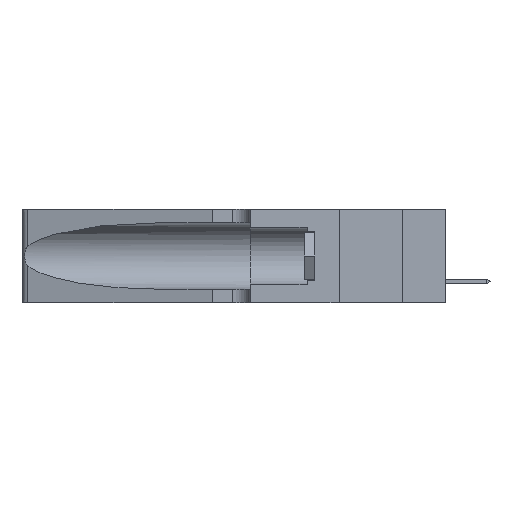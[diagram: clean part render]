
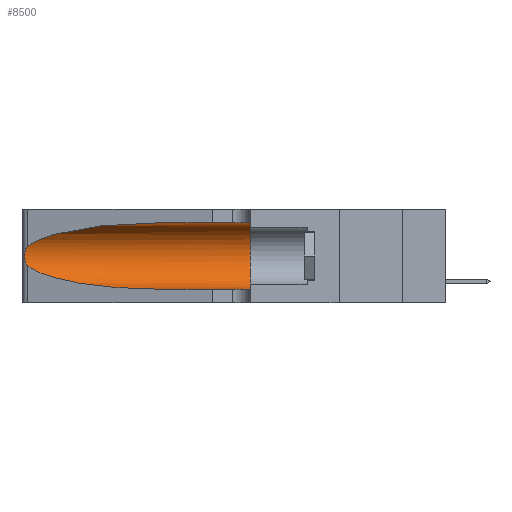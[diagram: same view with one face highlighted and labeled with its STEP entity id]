
A CAD part, left-side view. The second image highlights one B-rep face of the part: STEP entity #8500.
In plain terms, the highlighted cylindrical face has radius 3.308 mm (diameter 6.617 mm), a partial arc.
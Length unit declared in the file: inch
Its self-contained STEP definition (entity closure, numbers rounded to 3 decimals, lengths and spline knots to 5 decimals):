
#528 = ORIENTED_EDGE ( 'NONE', *, *, #15611, .F. ) ;
#548 = CARTESIAN_POINT ( 'NONE',  ( 0.1305, 1.61858, 0.185 ) ) ;
#616 = DIRECTION ( 'NONE',  ( 0., 0., -1. ) ) ;
#935 = CARTESIAN_POINT ( 'NONE',  ( 0.18966, 0.96281, 0.31525 ) ) ;
#961 = VECTOR ( 'NONE', #18069, 39.37008 ) ;
#1179 = CARTESIAN_POINT ( 'NONE',  ( 0.1305, 0.72297, 0.05475 ) ) ;
#1210 = AXIS2_PLACEMENT_3D ( 'NONE', #4689, #4761, #4612 ) ;
#1320 = CARTESIAN_POINT ( 'NONE',  ( 0.2373, 1.15595, 0.08982 ) ) ;
#1680 = CARTESIAN_POINT ( 'NONE',  ( 0.25487, 1.22718, 0.14631 ) ) ;
#1743 = VERTEX_POINT ( 'NONE', #8380 ) ;
#1961 = CARTESIAN_POINT ( 'NONE',  ( 0.25639, 1.23186, 0.15144 ) ) ;
#1983 = VERTEX_POINT ( 'NONE', #3956 ) ;
#2383 = B_SPLINE_CURVE_WITH_KNOTS ( 'NONE', 3,
 ( #12858, #4500, #4574, #17591, #7677, #8180, #15248, #16897, #18628, #20297, #18337, #1961, #13658, #1680 ),
 .UNSPECIFIED., .F., .F.,
 ( 4, 2, 2, 2, 2, 2, 4 ),
 ( 0., 0.00027, 0.00053, 0.00107, 0.0016, 0.00187, 0.00214 ),
 .UNSPECIFIED. ) ;
#2497 = VERTEX_POINT ( 'NONE', #15353 ) ;
#2686 = ORIENTED_EDGE ( 'NONE', *, *, #20262, .T. ) ;
#3001 = LINE ( 'NONE', #6966, #21076 ) ;
#3138 = ORIENTED_EDGE ( 'NONE', *, *, #20969, .T. ) ;
#3919 = ORIENTED_EDGE ( 'NONE', *, *, #8436, .F. ) ;
#3956 = CARTESIAN_POINT ( 'NONE',  ( 0.1305, 0.35, 0.31525 ) ) ;
#4019 = CIRCLE ( 'NONE', #1210, 0.13025 ) ;
#4206 = CARTESIAN_POINT ( 'NONE',  ( 0.25487, 1.22718, 0.22369 ) ) ;
#4500 = CARTESIAN_POINT ( 'NONE',  ( 0.25555, 1.22994, 0.2215 ) ) ;
#4574 = CARTESIAN_POINT ( 'NONE',  ( 0.25639, 1.23184, 0.21858 ) ) ;
#4578 = CARTESIAN_POINT ( 'NONE',  ( 0.18966, 0.96281, 0.05475 ) ) ;
#4612 = DIRECTION ( 'NONE',  ( 0., 0., 1. ) ) ;
#4689 = CARTESIAN_POINT ( 'NONE',  ( 0.1305, 0.35, 0.185 ) ) ;
#4761 = DIRECTION ( 'NONE',  ( 0., 1., 0. ) ) ;
#5115 = AXIS2_PLACEMENT_3D ( 'NONE', #548, #10481, #616 ) ;
#5933 = ORIENTED_EDGE ( 'NONE', *, *, #20416, .T. ) ;
#6376 = CARTESIAN_POINT ( 'NONE',  ( 0.1305, 1.61858, 0.05475 ) ) ;
#6966 = CARTESIAN_POINT ( 'NONE',  ( 0.1305, 1.61858, 0.31525 ) ) ;
#7677 = CARTESIAN_POINT ( 'NONE',  ( 0.25854, 1.2359, 0.20912 ) ) ;
#8180 = CARTESIAN_POINT ( 'NONE',  ( 0.26018, 1.23835, 0.19895 ) ) ;
#8380 = CARTESIAN_POINT ( 'NONE',  ( 0.1305, 0.72297, 0.31525 ) ) ;
#8436 = EDGE_CURVE ( 'NONE', #1743, #1983, #3001, .T. ) ;
#8500 = ADVANCED_FACE ( 'NONE', ( #20824 ), #12456, .F. ) ;
#10077 = EDGE_LOOP ( 'NONE', ( #5933, #17167, #3138, #2686, #528, #3919 ) ) ;
#10481 = DIRECTION ( 'NONE',  ( 0., -1., 0. ) ) ;
#11213 = VERTEX_POINT ( 'NONE', #20298 ) ;
#12456 = CYLINDRICAL_SURFACE ( 'NONE', #5115, 0.13025 ) ;
#12564 = CARTESIAN_POINT ( 'NONE',  ( 0.1305, 0.72297, 0.31525 ) ) ;
#12858 = CARTESIAN_POINT ( 'NONE',  ( 0.25487, 1.22718, 0.22369 ) ) ;
#12882 = VERTEX_POINT ( 'NONE', #14621 ) ;
#13658 = CARTESIAN_POINT ( 'NONE',  ( 0.25555, 1.22993, 0.14849 ) ) ;
#13800 = CARTESIAN_POINT ( 'NONE',  ( 0.2373, 1.15595, 0.28018 ) ) ;
#14621 = CARTESIAN_POINT ( 'NONE',  ( 0.1305, 0.35, 0.05475 ) ) ;
#15248 = CARTESIAN_POINT ( 'NONE',  ( 0.26075, 1.23896, 0.19203 ) ) ;
#15353 = CARTESIAN_POINT ( 'NONE',  ( 0.1305, 0.72297, 0.05475 ) ) ;
#15611 = EDGE_CURVE ( 'NONE', #1983, #12882, #4019, .T. ) ;
#16897 = CARTESIAN_POINT ( 'NONE',  ( 0.26075, 1.23896, 0.178 ) ) ;
#17167 = ORIENTED_EDGE ( 'NONE', *, *, #20375, .T. ) ;
#17591 = CARTESIAN_POINT ( 'NONE',  ( 0.25787, 1.23484, 0.2124 ) ) ;
#17627 =( BOUNDED_CURVE ( )  B_SPLINE_CURVE ( 3, ( #17824, #1320, #4578, #1179 ),
 .UNSPECIFIED., .F., .T. ) 
 B_SPLINE_CURVE_WITH_KNOTS ( ( 4, 4 ),
 ( 3.44316, 4.71239 ),
 .UNSPECIFIED. ) 
 CURVE ( )  GEOMETRIC_REPRESENTATION_ITEM ( )  RATIONAL_B_SPLINE_CURVE ( ( 1., 0.87, 0.87, 1. ) ) 
 REPRESENTATION_ITEM ( '' )  );
#17716 = CARTESIAN_POINT ( 'NONE',  ( 0.25487, 1.22718, 0.22369 ) ) ;
#17824 = CARTESIAN_POINT ( 'NONE',  ( 0.25487, 1.22718, 0.14631 ) ) ;
#18069 = DIRECTION ( 'NONE',  ( 0., -1., 0. ) ) ;
#18337 = CARTESIAN_POINT ( 'NONE',  ( 0.25789, 1.23486, 0.15765 ) ) ;
#18628 = CARTESIAN_POINT ( 'NONE',  ( 0.26017, 1.23833, 0.17102 ) ) ;
#18663 = DIRECTION ( 'NONE',  ( 0., -1., 0. ) ) ;
#20262 = EDGE_CURVE ( 'NONE', #2497, #12882, #20855, .T. ) ;
#20297 = CARTESIAN_POINT ( 'NONE',  ( 0.25856, 1.23593, 0.16098 ) ) ;
#20298 = CARTESIAN_POINT ( 'NONE',  ( 0.25487, 1.22718, 0.14631 ) ) ;
#20375 = EDGE_CURVE ( 'NONE', #21507, #11213, #2383, .T. ) ;
#20416 = EDGE_CURVE ( 'NONE', #1743, #21507, #21558, .T. ) ;
#20824 = FACE_OUTER_BOUND ( 'NONE', #10077, .T. ) ;
#20855 = LINE ( 'NONE', #6376, #961 ) ;
#20969 = EDGE_CURVE ( 'NONE', #11213, #2497, #17627, .T. ) ;
#21076 = VECTOR ( 'NONE', #18663, 39.37008 ) ;
#21507 = VERTEX_POINT ( 'NONE', #17716 ) ;
#21558 =( BOUNDED_CURVE ( )  B_SPLINE_CURVE ( 3, ( #12564, #935, #13800, #4206 ),
 .UNSPECIFIED., .F., .F. ) 
 B_SPLINE_CURVE_WITH_KNOTS ( ( 4, 4 ),
 ( 1.5708, 2.84003 ),
 .UNSPECIFIED. ) 
 CURVE ( )  GEOMETRIC_REPRESENTATION_ITEM ( )  RATIONAL_B_SPLINE_CURVE ( ( 1., 0.87, 0.87, 1. ) ) 
 REPRESENTATION_ITEM ( '' )  );
